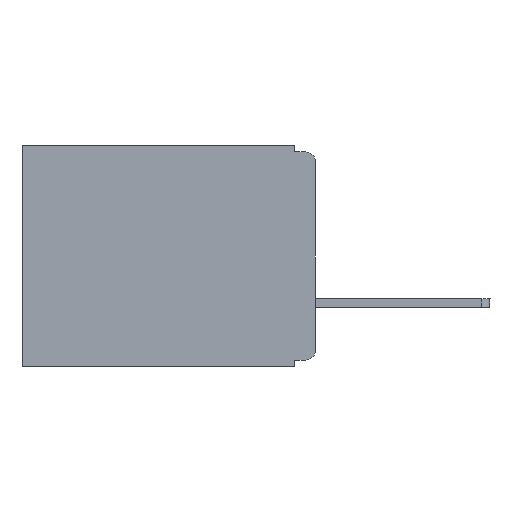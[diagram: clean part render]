
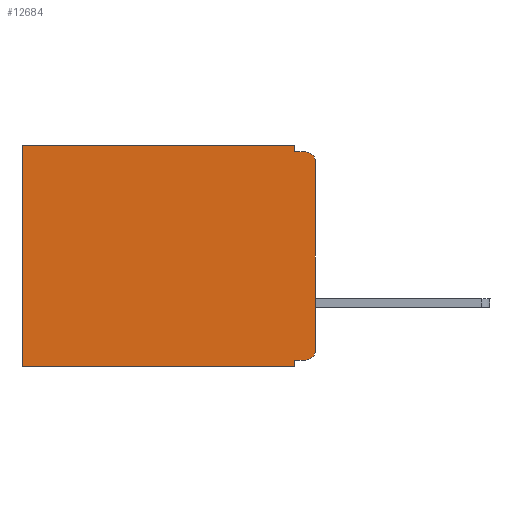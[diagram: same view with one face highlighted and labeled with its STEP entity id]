
A CAD part, left-side view. The second image highlights one B-rep face of the part: STEP entity #12684.
In plain terms, the highlighted planar face has unit normal (-1, 0, 0).
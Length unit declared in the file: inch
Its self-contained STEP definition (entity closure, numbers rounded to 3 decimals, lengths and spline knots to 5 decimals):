
#31 = CARTESIAN_POINT ( 'NONE',  ( 0.3, 0.031, -0.01 ) ) ;
#59 = DIRECTION ( 'NONE',  ( 0., 0., -1. ) ) ;
#110 = VECTOR ( 'NONE', #13767, 39.37008 ) ;
#448 = ORIENTED_EDGE ( 'NONE', *, *, #7115, .F. ) ;
#638 = AXIS2_PLACEMENT_3D ( 'NONE', #12016, #5169, #6413 ) ;
#672 = CARTESIAN_POINT ( 'NONE',  ( 0.3, 0.015, -0.32 ) ) ;
#1097 = VERTEX_POINT ( 'NONE', #6756 ) ;
#1242 = ORIENTED_EDGE ( 'NONE', *, *, #9918, .T. ) ;
#1348 = EDGE_CURVE ( 'NONE', #1729, #3043, #4534, .T. ) ;
#1470 = LINE ( 'NONE', #12420, #6565 ) ;
#1554 = VERTEX_POINT ( 'NONE', #672 ) ;
#1675 = ORIENTED_EDGE ( 'NONE', *, *, #8527, .T. ) ;
#1729 = VERTEX_POINT ( 'NONE', #2197 ) ;
#1814 = VERTEX_POINT ( 'NONE', #13732 ) ;
#2042 = CARTESIAN_POINT ( 'NONE',  ( 0.3, 0.015, -0.305 ) ) ;
#2197 = CARTESIAN_POINT ( 'NONE',  ( 0.3, 0., -0.025 ) ) ;
#2620 = LINE ( 'NONE', #4653, #110 ) ;
#2653 = DIRECTION ( 'NONE',  ( 0., 0., -1. ) ) ;
#2666 = ORIENTED_EDGE ( 'NONE', *, *, #13418, .F. ) ;
#3020 = CARTESIAN_POINT ( 'NONE',  ( 0.3, 0.031, 0. ) ) ;
#3043 = VERTEX_POINT ( 'NONE', #3302 ) ;
#3302 = CARTESIAN_POINT ( 'NONE',  ( 0.3, 0.015, -0.01 ) ) ;
#3361 = ORIENTED_EDGE ( 'NONE', *, *, #11084, .F. ) ;
#3586 = VECTOR ( 'NONE', #3703, 39.37008 ) ;
#3703 = DIRECTION ( 'NONE',  ( 0., 0., -1. ) ) ;
#3734 = CIRCLE ( 'NONE', #9323, 0.015 ) ;
#3753 = CARTESIAN_POINT ( 'NONE',  ( 0.3, 0.437, 0. ) ) ;
#4497 = DIRECTION ( 'NONE',  ( 0., 0., -1. ) ) ;
#4534 = CIRCLE ( 'NONE', #4548, 0.015 ) ;
#4548 = AXIS2_PLACEMENT_3D ( 'NONE', #6020, #11629, #2653 ) ;
#4572 = CARTESIAN_POINT ( 'NONE',  ( 0.3, 0., 0. ) ) ;
#4653 = CARTESIAN_POINT ( 'NONE',  ( 0.3, 0., -0.32 ) ) ;
#4662 = CARTESIAN_POINT ( 'NONE',  ( 0.3, 0., -0.01 ) ) ;
#4785 = CARTESIAN_POINT ( 'NONE',  ( 0.3, 0., -0.33 ) ) ;
#4852 = LINE ( 'NONE', #11282, #6086 ) ;
#5169 = DIRECTION ( 'NONE',  ( 1., 0., 0. ) ) ;
#5534 = DIRECTION ( 'NONE',  ( 0., 0., -1. ) ) ;
#6020 = CARTESIAN_POINT ( 'NONE',  ( 0.3, 0.015, -0.025 ) ) ;
#6086 = VECTOR ( 'NONE', #4497, 39.37008 ) ;
#6243 = EDGE_CURVE ( 'NONE', #1554, #7021, #2620, .T. ) ;
#6315 = ORIENTED_EDGE ( 'NONE', *, *, #8829, .T. ) ;
#6413 = DIRECTION ( 'NONE',  ( 0., 0., -1. ) ) ;
#6462 = PLANE ( 'NONE',  #638 ) ;
#6565 = VECTOR ( 'NONE', #5534, 39.37008 ) ;
#6756 = CARTESIAN_POINT ( 'NONE',  ( 0.3, 0.031, -0.33 ) ) ;
#6906 = LINE ( 'NONE', #4572, #9069 ) ;
#7021 = VERTEX_POINT ( 'NONE', #10329 ) ;
#7064 = CARTESIAN_POINT ( 'NONE',  ( 0.3, 0.031, -0.33 ) ) ;
#7115 = EDGE_CURVE ( 'NONE', #1097, #1814, #13746, .T. ) ;
#8081 = EDGE_CURVE ( 'NONE', #7021, #1097, #8924, .T. ) ;
#8527 = EDGE_CURVE ( 'NONE', #13614, #1814, #1470, .T. ) ;
#8668 = LINE ( 'NONE', #12519, #14200 ) ;
#8801 = FACE_OUTER_BOUND ( 'NONE', #11325, .T. ) ;
#8809 = VERTEX_POINT ( 'NONE', #14242 ) ;
#8829 = EDGE_CURVE ( 'NONE', #1554, #8809, #3734, .T. ) ;
#8924 = LINE ( 'NONE', #7064, #3586 ) ;
#9030 = LINE ( 'NONE', #4662, #10983 ) ;
#9069 = VECTOR ( 'NONE', #9265, 39.37008 ) ;
#9265 = DIRECTION ( 'NONE',  ( 0., 1., 0. ) ) ;
#9323 = AXIS2_PLACEMENT_3D ( 'NONE', #2042, #9866, #14488 ) ;
#9866 = DIRECTION ( 'NONE',  ( -1., 0., 0. ) ) ;
#9918 = EDGE_CURVE ( 'NONE', #14309, #13614, #6906, .T. ) ;
#10254 = ORIENTED_EDGE ( 'NONE', *, *, #11729, .F. ) ;
#10329 = CARTESIAN_POINT ( 'NONE',  ( 0.3, 0.031, -0.32 ) ) ;
#10715 = VERTEX_POINT ( 'NONE', #31 ) ;
#10983 = VECTOR ( 'NONE', #12636, 39.37008 ) ;
#11084 = EDGE_CURVE ( 'NONE', #1729, #8809, #8668, .T. ) ;
#11282 = CARTESIAN_POINT ( 'NONE',  ( 0.3, 0.031, 0. ) ) ;
#11325 = EDGE_LOOP ( 'NONE', ( #3361, #12909, #10254, #2666, #1242, #1675, #448, #11905, #13794, #6315 ) ) ;
#11629 = DIRECTION ( 'NONE',  ( -1., 0., 0. ) ) ;
#11729 = EDGE_CURVE ( 'NONE', #10715, #3043, #9030, .T. ) ;
#11905 = ORIENTED_EDGE ( 'NONE', *, *, #8081, .F. ) ;
#12016 = CARTESIAN_POINT ( 'NONE',  ( 0.3, 0., -0.33 ) ) ;
#12420 = CARTESIAN_POINT ( 'NONE',  ( 0.3, 0.437, -0.33 ) ) ;
#12505 = VECTOR ( 'NONE', #13910, 39.37008 ) ;
#12519 = CARTESIAN_POINT ( 'NONE',  ( 0.3, 0., -0.33 ) ) ;
#12636 = DIRECTION ( 'NONE',  ( 0., -1., 0. ) ) ;
#12684 = ADVANCED_FACE ( 'NONE', ( #8801 ), #6462, .F. ) ;
#12909 = ORIENTED_EDGE ( 'NONE', *, *, #1348, .T. ) ;
#13418 = EDGE_CURVE ( 'NONE', #14309, #10715, #4852, .T. ) ;
#13614 = VERTEX_POINT ( 'NONE', #3753 ) ;
#13732 = CARTESIAN_POINT ( 'NONE',  ( 0.3, 0.437, -0.33 ) ) ;
#13746 = LINE ( 'NONE', #4785, #12505 ) ;
#13767 = DIRECTION ( 'NONE',  ( 0., 1., 0. ) ) ;
#13794 = ORIENTED_EDGE ( 'NONE', *, *, #6243, .F. ) ;
#13910 = DIRECTION ( 'NONE',  ( 0., 1., 0. ) ) ;
#14200 = VECTOR ( 'NONE', #59, 39.37008 ) ;
#14242 = CARTESIAN_POINT ( 'NONE',  ( 0.3, 0., -0.305 ) ) ;
#14309 = VERTEX_POINT ( 'NONE', #3020 ) ;
#14488 = DIRECTION ( 'NONE',  ( 0., 0., -1. ) ) ;
